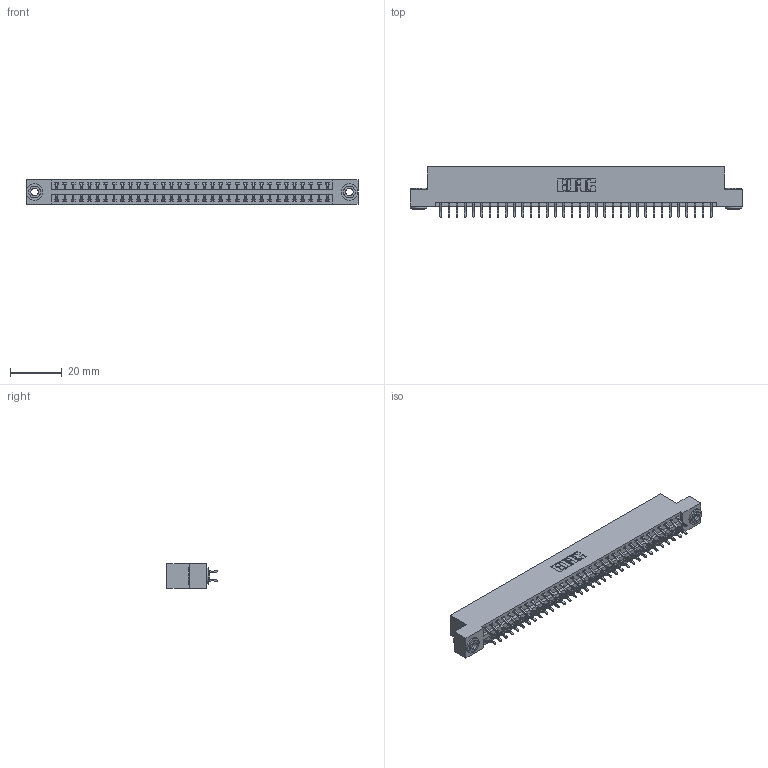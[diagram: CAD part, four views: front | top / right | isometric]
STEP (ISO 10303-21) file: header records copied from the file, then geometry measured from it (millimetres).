
FILE_DESCRIPTION (( 'STEP AP203' ), '1' );
FILE_NAME ('396-068-556-203.STEP', '2019-10-30T19:03:48', ( '' ), ( '' ), 'SwSTEP 2.0', 'SolidWorks 2016', '' );
FILE_SCHEMA (( 'CONFIG_CONTROL_DESIGN' ));
Length unit declared in the file: inch
Products named in the file (4): 345-250-002_345-250-002-102; 396-068-556-203; 346 Part_Flush Mounting Lugs - 0.156 Dia-TH; 345-292-001_556 Tail
Assembly tree (71 placements, depth 2):
  396-068-556-203
    346 Part_Flush Mounting Lugs - 0.156 Dia-TH
    345-292-001_556 Tail  x68
    345-250-002_345-250-002-102  x2
Bounding box: 128.52 x 19.57 x 9.4 mm (x, y, z)
Volume: 12487.3 mm3; surface area: 17189.8 mm2
Topology: 71 solids, 71 shells, 4104 faces, 12169 edges, 8018 vertices
Faces by surface type: plane 2738, cylinder 1358, cone 8
Entity records: 24136 total; most frequent: CARTESIAN_POINT 3979, ORIENTED_EDGE 3894, DIRECTION 3577, EDGE_CURVE 1947, LINE 1647, VECTOR 1647, VERTEX_POINT 1294, AXIS2_PLACEMENT_3D 965
